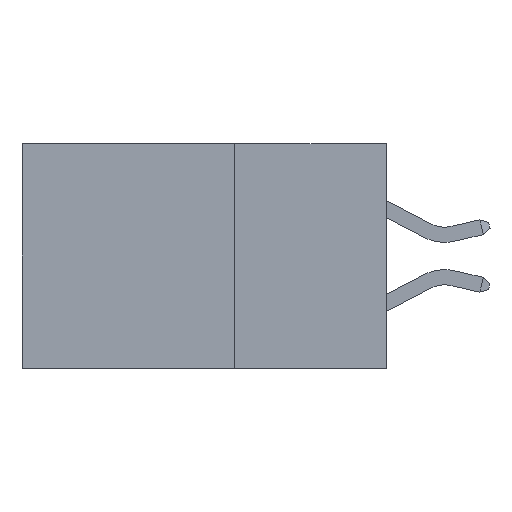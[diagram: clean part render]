
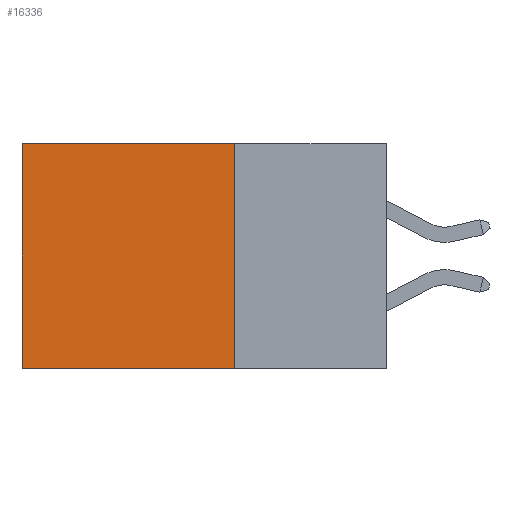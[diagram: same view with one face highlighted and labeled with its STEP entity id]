
A CAD part, left-side view. The second image highlights one B-rep face of the part: STEP entity #16336.
In plain terms, the highlighted planar face has unit normal (-1, 0, 0).
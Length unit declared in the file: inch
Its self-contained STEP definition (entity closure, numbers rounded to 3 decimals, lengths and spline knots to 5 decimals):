
#1038 = AXIS2_PLACEMENT_3D ( 'NONE', #22370, #24512, #11512 ) ;
#2674 = PLANE ( 'NONE',  #1038 ) ;
#3624 = EDGE_LOOP ( 'NONE', ( #8221, #20734, #8358, #10760 ) ) ;
#3829 = DIRECTION ( 'NONE',  ( 0., 1., 0. ) ) ;
#5108 = CARTESIAN_POINT ( 'NONE',  ( 0.298, 0.6, 0. ) ) ;
#6736 = CARTESIAN_POINT ( 'NONE',  ( 0.298, 0.6, 0. ) ) ;
#6906 = FACE_OUTER_BOUND ( 'NONE', #3624, .T. ) ;
#7147 = CARTESIAN_POINT ( 'NONE',  ( 0.298, 0.25, 0. ) ) ;
#7454 = CARTESIAN_POINT ( 'NONE',  ( 0.298, 0.6, -0.37 ) ) ;
#8125 = CARTESIAN_POINT ( 'NONE',  ( 0.298, 0.25, 0. ) ) ;
#8221 = ORIENTED_EDGE ( 'NONE', *, *, #20031, .T. ) ;
#8358 = ORIENTED_EDGE ( 'NONE', *, *, #14451, .F. ) ;
#8792 = VERTEX_POINT ( 'NONE', #7147 ) ;
#8913 = VERTEX_POINT ( 'NONE', #12010 ) ;
#9102 = CARTESIAN_POINT ( 'NONE',  ( 0.298, 0.25, -0.37 ) ) ;
#10172 = VECTOR ( 'NONE', #19807, 39.37008 ) ;
#10266 = VERTEX_POINT ( 'NONE', #7454 ) ;
#10760 = ORIENTED_EDGE ( 'NONE', *, *, #18544, .T. ) ;
#11196 = VECTOR ( 'NONE', #3829, 39.37008 ) ;
#11283 = DIRECTION ( 'NONE',  ( 0., 1., 0. ) ) ;
#11512 = DIRECTION ( 'NONE',  ( 0., 0., -1. ) ) ;
#12010 = CARTESIAN_POINT ( 'NONE',  ( 0.298, 0.25, -0.37 ) ) ;
#14087 = EDGE_CURVE ( 'NONE', #8913, #10266, #26400, .T. ) ;
#14249 = VECTOR ( 'NONE', #11283, 39.37008 ) ;
#14451 = EDGE_CURVE ( 'NONE', #8792, #8913, #22033, .T. ) ;
#16336 = ADVANCED_FACE ( 'NONE', ( #6906 ), #2674, .F. ) ;
#16997 = LINE ( 'NONE', #19098, #11196 ) ;
#17030 = VERTEX_POINT ( 'NONE', #5108 ) ;
#18544 = EDGE_CURVE ( 'NONE', #8792, #17030, #16997, .T. ) ;
#19080 = DIRECTION ( 'NONE',  ( 0., 0., -1. ) ) ;
#19098 = CARTESIAN_POINT ( 'NONE',  ( 0.298, 0.25, 0. ) ) ;
#19807 = DIRECTION ( 'NONE',  ( 0., 0., -1. ) ) ;
#20031 = EDGE_CURVE ( 'NONE', #17030, #10266, #27442, .T. ) ;
#20734 = ORIENTED_EDGE ( 'NONE', *, *, #14087, .F. ) ;
#22033 = LINE ( 'NONE', #8125, #27659 ) ;
#22370 = CARTESIAN_POINT ( 'NONE',  ( 0.298, 0.25, 0. ) ) ;
#24512 = DIRECTION ( 'NONE',  ( 1., 0., 0. ) ) ;
#26400 = LINE ( 'NONE', #9102, #14249 ) ;
#27442 = LINE ( 'NONE', #6736, #10172 ) ;
#27659 = VECTOR ( 'NONE', #19080, 39.37008 ) ;
